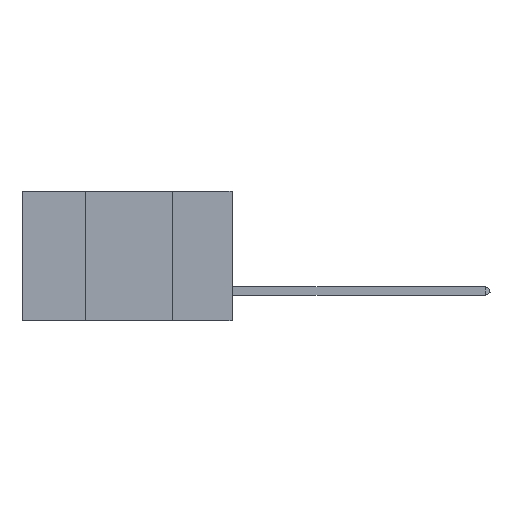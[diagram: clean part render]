
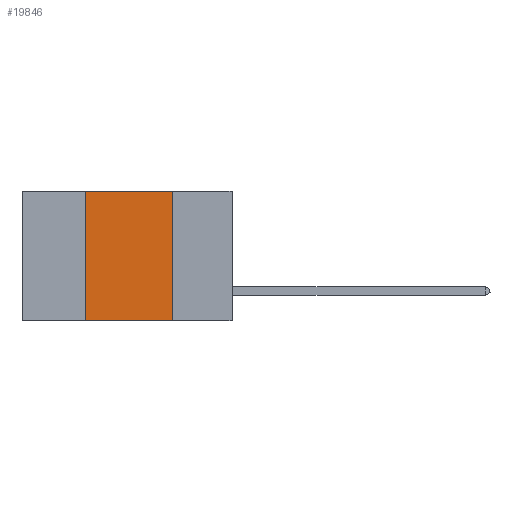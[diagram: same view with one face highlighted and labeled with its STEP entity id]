
A CAD part, left-side view. The second image highlights one B-rep face of the part: STEP entity #19846.
In plain terms, the highlighted planar face has unit normal (-1, 0, 0).
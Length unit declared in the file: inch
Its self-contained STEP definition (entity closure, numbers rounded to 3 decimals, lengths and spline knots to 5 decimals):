
#106 = ORIENTED_EDGE ( 'NONE', *, *, #3322, .F. ) ;
#463 = CARTESIAN_POINT ( 'NONE',  ( 0., 0.17, 0. ) ) ;
#757 = DIRECTION ( 'NONE',  ( 0., 0., -1. ) ) ;
#1619 = CARTESIAN_POINT ( 'NONE',  ( 0., 0.42, 0. ) ) ;
#1917 = DIRECTION ( 'NONE',  ( 0., 0., 1. ) ) ;
#3322 = EDGE_CURVE ( 'NONE', #10252, #18434, #18329, .T. ) ;
#3799 = CARTESIAN_POINT ( 'NONE',  ( 0., 0.42, -0.37 ) ) ;
#4679 = VECTOR ( 'NONE', #8353, 39.37008 ) ;
#5133 = EDGE_CURVE ( 'NONE', #10252, #7703, #12922, .T. ) ;
#6536 = CARTESIAN_POINT ( 'NONE',  ( 0., 0.17, -0.37 ) ) ;
#7411 = FACE_OUTER_BOUND ( 'NONE', #17732, .T. ) ;
#7703 = VERTEX_POINT ( 'NONE', #6536 ) ;
#8353 = DIRECTION ( 'NONE',  ( 0., -1., 0. ) ) ;
#10069 = EDGE_CURVE ( 'NONE', #18434, #18744, #17218, .T. ) ;
#10252 = VERTEX_POINT ( 'NONE', #3799 ) ;
#10541 = CARTESIAN_POINT ( 'NONE',  ( 0., 0.17, 0. ) ) ;
#10971 = VECTOR ( 'NONE', #757, 39.37008 ) ;
#11796 = CARTESIAN_POINT ( 'NONE',  ( 0., 0.6, 0. ) ) ;
#12215 = VECTOR ( 'NONE', #1917, 39.37008 ) ;
#12922 = LINE ( 'NONE', #14377, #17274 ) ;
#13497 = PLANE ( 'NONE',  #15050 ) ;
#13656 = ORIENTED_EDGE ( 'NONE', *, *, #5133, .T. ) ;
#14241 = ORIENTED_EDGE ( 'NONE', *, *, #14378, .F. ) ;
#14377 = CARTESIAN_POINT ( 'NONE',  ( 0., 0.6, -0.37 ) ) ;
#14378 = EDGE_CURVE ( 'NONE', #18744, #7703, #15327, .T. ) ;
#14932 = DIRECTION ( 'NONE',  ( 1., 0., 0. ) ) ;
#15050 = AXIS2_PLACEMENT_3D ( 'NONE', #11796, #14932, #15068 ) ;
#15068 = DIRECTION ( 'NONE',  ( 0., 0., -1. ) ) ;
#15327 = LINE ( 'NONE', #10541, #10971 ) ;
#16170 = DIRECTION ( 'NONE',  ( 0., -1., 0. ) ) ;
#16468 = CARTESIAN_POINT ( 'NONE',  ( 0., 0.6, 0. ) ) ;
#17218 = LINE ( 'NONE', #16468, #4679 ) ;
#17274 = VECTOR ( 'NONE', #16170, 39.37008 ) ;
#17689 = CARTESIAN_POINT ( 'NONE',  ( 0., 0.42, 0. ) ) ;
#17732 = EDGE_LOOP ( 'NONE', ( #14241, #19594, #106, #13656 ) ) ;
#18329 = LINE ( 'NONE', #1619, #12215 ) ;
#18434 = VERTEX_POINT ( 'NONE', #17689 ) ;
#18744 = VERTEX_POINT ( 'NONE', #463 ) ;
#19594 = ORIENTED_EDGE ( 'NONE', *, *, #10069, .F. ) ;
#19846 = ADVANCED_FACE ( 'NONE', ( #7411 ), #13497, .F. ) ;
